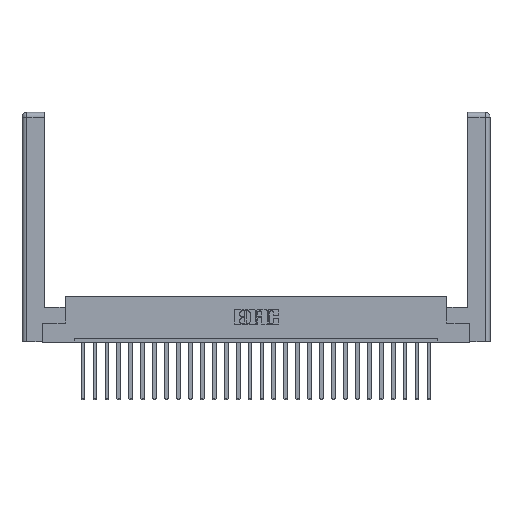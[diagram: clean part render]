
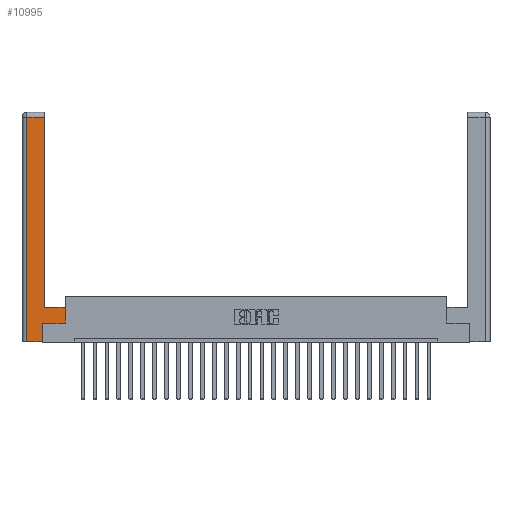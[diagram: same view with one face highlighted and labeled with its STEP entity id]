
A CAD part, top view. The second image highlights one B-rep face of the part: STEP entity #10995.
In plain terms, the highlighted planar face has unit normal (0, 0, 1).
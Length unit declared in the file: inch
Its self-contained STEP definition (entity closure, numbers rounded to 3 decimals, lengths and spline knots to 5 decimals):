
#21 = DIRECTION ( 'NONE',  ( 1., 0., 0. ) ) ;
#186 = VECTOR ( 'NONE', #7362, 39.37008 ) ;
#246 = DIRECTION ( 'NONE',  ( 0., 1., 0. ) ) ;
#268 = DIRECTION ( 'NONE',  ( 1., 0., 0. ) ) ;
#582 = CARTESIAN_POINT ( 'NONE',  ( 0.265, 0.245, 0. ) ) ;
#801 = ORIENTED_EDGE ( 'NONE', *, *, #2194, .T. ) ;
#832 = DIRECTION ( 'NONE',  ( -1., 0., 0. ) ) ;
#1505 = VERTEX_POINT ( 'NONE', #15869 ) ;
#2194 = EDGE_CURVE ( 'NONE', #1505, #6781, #24499, .T. ) ;
#2227 = ORIENTED_EDGE ( 'NONE', *, *, #24228, .T. ) ;
#2693 = VERTEX_POINT ( 'NONE', #21986 ) ;
#3479 = ORIENTED_EDGE ( 'NONE', *, *, #15241, .T. ) ;
#3505 = EDGE_CURVE ( 'NONE', #2693, #22024, #12315, .T. ) ;
#4273 = CARTESIAN_POINT ( 'NONE',  ( 0.565, 0.245, 0. ) ) ;
#4609 = ORIENTED_EDGE ( 'NONE', *, *, #3505, .T. ) ;
#4733 = PLANE ( 'NONE',  #25723 ) ;
#4820 = DIRECTION ( 'NONE',  ( 0., 0., -1. ) ) ;
#4830 = DIRECTION ( 'NONE',  ( 0., 1., 0. ) ) ;
#6619 = VERTEX_POINT ( 'NONE', #19379 ) ;
#6781 = VERTEX_POINT ( 'NONE', #24559 ) ;
#7008 = VERTEX_POINT ( 'NONE', #7080 ) ;
#7080 = CARTESIAN_POINT ( 'NONE',  ( 0.565, 0.245, 0. ) ) ;
#7362 = DIRECTION ( 'NONE',  ( -1., 0., 0. ) ) ;
#7746 = CARTESIAN_POINT ( 'NONE',  ( 0.265, 0., 0. ) ) ;
#8025 = CARTESIAN_POINT ( 'NONE',  ( 0.265, 0.245, 0. ) ) ;
#8140 = LINE ( 'NONE', #9302, #186 ) ;
#8665 = VERTEX_POINT ( 'NONE', #582 ) ;
#9190 = EDGE_CURVE ( 'NONE', #8665, #7008, #13347, .T. ) ;
#9302 = CARTESIAN_POINT ( 'NONE',  ( 0.0615, 2.94, 0. ) ) ;
#9426 = LINE ( 'NONE', #19902, #18340 ) ;
#9746 = EDGE_CURVE ( 'NONE', #7008, #6619, #11103, .T. ) ;
#10483 = ORIENTED_EDGE ( 'NONE', *, *, #9746, .T. ) ;
#10716 = DIRECTION ( 'NONE',  ( 0., 1., 0. ) ) ;
#10995 = ADVANCED_FACE ( 'NONE', ( #12164 ), #4733, .F. ) ;
#11103 = LINE ( 'NONE', #25052, #14600 ) ;
#11812 = DIRECTION ( 'NONE',  ( 0., -1., 0. ) ) ;
#11882 = DIRECTION ( 'NONE',  ( -1., 0., 0. ) ) ;
#12164 = FACE_OUTER_BOUND ( 'NONE', #26291, .T. ) ;
#12315 = LINE ( 'NONE', #13834, #24738 ) ;
#12606 = VECTOR ( 'NONE', #246, 39.37008 ) ;
#12653 = CARTESIAN_POINT ( 'NONE',  ( 0.0615, 2.94, 0. ) ) ;
#12707 = CARTESIAN_POINT ( 'NONE',  ( 0., 0., 0. ) ) ;
#13346 = ORIENTED_EDGE ( 'NONE', *, *, #23538, .T. ) ;
#13347 = LINE ( 'NONE', #4273, #14309 ) ;
#13834 = CARTESIAN_POINT ( 'NONE',  ( 0.265, 0., 0. ) ) ;
#14309 = VECTOR ( 'NONE', #268, 39.37008 ) ;
#14351 = EDGE_CURVE ( 'NONE', #17756, #2693, #9426, .T. ) ;
#14600 = VECTOR ( 'NONE', #10716, 39.37008 ) ;
#15241 = EDGE_CURVE ( 'NONE', #6619, #1505, #17638, .T. ) ;
#15869 = CARTESIAN_POINT ( 'NONE',  ( 0.295, 0.45, 0. ) ) ;
#15977 = ORIENTED_EDGE ( 'NONE', *, *, #14351, .T. ) ;
#16112 = CARTESIAN_POINT ( 'NONE',  ( 0.295, 0.45, 0. ) ) ;
#16941 = CARTESIAN_POINT ( 'NONE',  ( 0.295, 3., 0. ) ) ;
#17638 = LINE ( 'NONE', #16112, #24370 ) ;
#17756 = VERTEX_POINT ( 'NONE', #12653 ) ;
#17970 = LINE ( 'NONE', #8025, #12606 ) ;
#18340 = VECTOR ( 'NONE', #11812, 39.37008 ) ;
#18401 = ORIENTED_EDGE ( 'NONE', *, *, #9190, .T. ) ;
#19379 = CARTESIAN_POINT ( 'NONE',  ( 0.565, 0.45, 0. ) ) ;
#19902 = CARTESIAN_POINT ( 'NONE',  ( 0.0615, 0., 0. ) ) ;
#20978 = VECTOR ( 'NONE', #4830, 39.37008 ) ;
#21986 = CARTESIAN_POINT ( 'NONE',  ( 0.0615, 0., 0. ) ) ;
#22024 = VERTEX_POINT ( 'NONE', #7746 ) ;
#23538 = EDGE_CURVE ( 'NONE', #22024, #8665, #17970, .T. ) ;
#24228 = EDGE_CURVE ( 'NONE', #6781, #17756, #8140, .T. ) ;
#24370 = VECTOR ( 'NONE', #11882, 39.37008 ) ;
#24499 = LINE ( 'NONE', #16941, #20978 ) ;
#24559 = CARTESIAN_POINT ( 'NONE',  ( 0.295, 2.94, 0. ) ) ;
#24738 = VECTOR ( 'NONE', #21, 39.37008 ) ;
#25052 = CARTESIAN_POINT ( 'NONE',  ( 0.565, 0.45, 0. ) ) ;
#25723 = AXIS2_PLACEMENT_3D ( 'NONE', #12707, #4820, #832 ) ;
#26291 = EDGE_LOOP ( 'NONE', ( #801, #2227, #15977, #4609, #13346, #18401, #10483, #3479 ) ) ;
